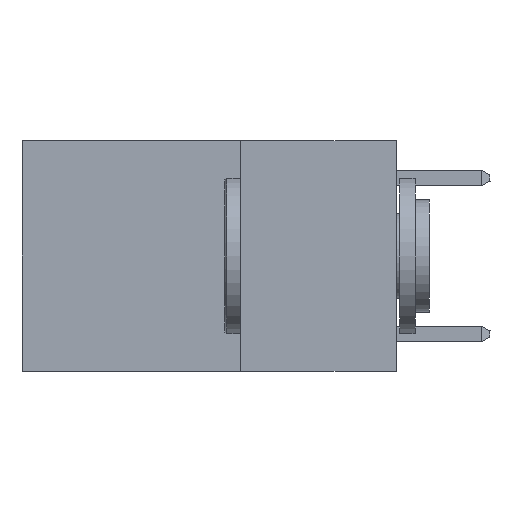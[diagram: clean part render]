
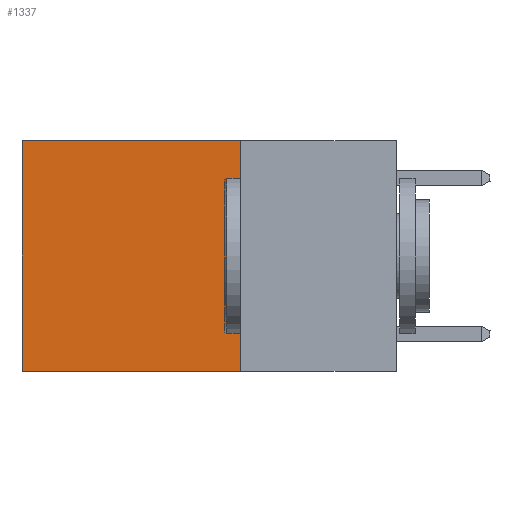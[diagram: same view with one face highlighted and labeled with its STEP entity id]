
A CAD part, left-side view. The second image highlights one B-rep face of the part: STEP entity #1337.
In plain terms, the highlighted planar face has unit normal (-1, 0, 0).
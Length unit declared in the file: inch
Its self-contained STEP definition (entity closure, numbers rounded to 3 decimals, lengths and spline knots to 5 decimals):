
#533 = CARTESIAN_POINT ( 'NONE',  ( 0.2625, 0.25, -0.37 ) ) ;
#821 = FACE_OUTER_BOUND ( 'NONE', #13358, .T. ) ;
#1337 = ADVANCED_FACE ( 'NONE', ( #821 ), #2096, .F. ) ;
#1387 = CARTESIAN_POINT ( 'NONE',  ( 0.2625, 0.6, 0. ) ) ;
#1542 = CARTESIAN_POINT ( 'NONE',  ( 0.2625, 0.25, 0. ) ) ;
#2096 = PLANE ( 'NONE',  #23755 ) ;
#2467 = ORIENTED_EDGE ( 'NONE', *, *, #15455, .F. ) ;
#4853 = CARTESIAN_POINT ( 'NONE',  ( 0.2625, 0.6, 0. ) ) ;
#5126 = EDGE_CURVE ( 'NONE', #6760, #14929, #12306, .T. ) ;
#6651 = ORIENTED_EDGE ( 'NONE', *, *, #13744, .T. ) ;
#6760 = VERTEX_POINT ( 'NONE', #11339 ) ;
#7206 = CARTESIAN_POINT ( 'NONE',  ( 0.2625, 0.25, 0. ) ) ;
#9534 = DIRECTION ( 'NONE',  ( 0., 0., -1. ) ) ;
#9906 = ORIENTED_EDGE ( 'NONE', *, *, #28513, .T. ) ;
#11339 = CARTESIAN_POINT ( 'NONE',  ( 0.2625, 0.25, -0.37 ) ) ;
#12306 = LINE ( 'NONE', #533, #28080 ) ;
#12345 = ORIENTED_EDGE ( 'NONE', *, *, #5126, .F. ) ;
#12753 = DIRECTION ( 'NONE',  ( 0., 1., 0. ) ) ;
#13343 = LINE ( 'NONE', #22816, #22831 ) ;
#13358 = EDGE_LOOP ( 'NONE', ( #9906, #12345, #2467, #6651 ) ) ;
#13744 = EDGE_CURVE ( 'NONE', #18459, #20859, #13343, .T. ) ;
#14929 = VERTEX_POINT ( 'NONE', #24857 ) ;
#15455 = EDGE_CURVE ( 'NONE', #18459, #6760, #16106, .T. ) ;
#16106 = LINE ( 'NONE', #1542, #21953 ) ;
#18459 = VERTEX_POINT ( 'NONE', #20870 ) ;
#18836 = DIRECTION ( 'NONE',  ( 1., 0., 0. ) ) ;
#20448 = DIRECTION ( 'NONE',  ( 0., 0., -1. ) ) ;
#20456 = DIRECTION ( 'NONE',  ( 0., 0., -1. ) ) ;
#20859 = VERTEX_POINT ( 'NONE', #4853 ) ;
#20870 = CARTESIAN_POINT ( 'NONE',  ( 0.2625, 0.25, 0. ) ) ;
#21953 = VECTOR ( 'NONE', #20456, 39.37008 ) ;
#22816 = CARTESIAN_POINT ( 'NONE',  ( 0.2625, 0.25, 0. ) ) ;
#22831 = VECTOR ( 'NONE', #24048, 39.37008 ) ;
#23755 = AXIS2_PLACEMENT_3D ( 'NONE', #7206, #18836, #9534 ) ;
#23985 = VECTOR ( 'NONE', #20448, 39.37008 ) ;
#24048 = DIRECTION ( 'NONE',  ( 0., 1., 0. ) ) ;
#24857 = CARTESIAN_POINT ( 'NONE',  ( 0.2625, 0.6, -0.37 ) ) ;
#24965 = LINE ( 'NONE', #1387, #23985 ) ;
#28080 = VECTOR ( 'NONE', #12753, 39.37008 ) ;
#28513 = EDGE_CURVE ( 'NONE', #20859, #14929, #24965, .T. ) ;
